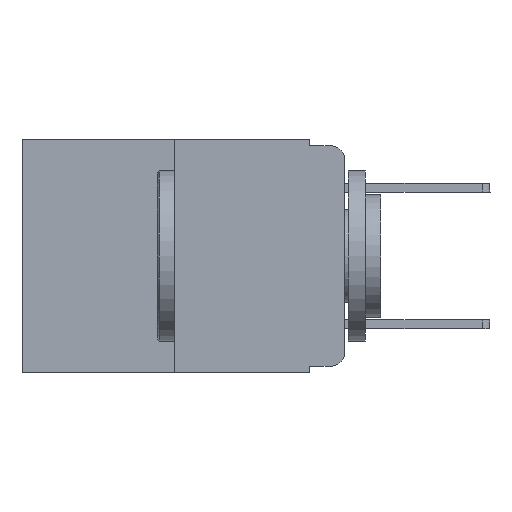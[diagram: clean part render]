
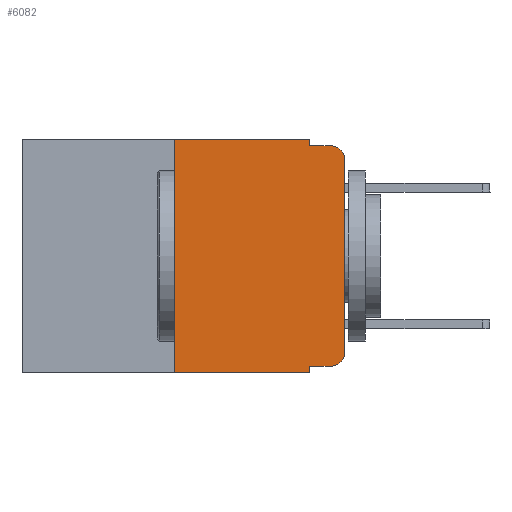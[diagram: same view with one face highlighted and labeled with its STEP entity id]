
A CAD part, left-side view. The second image highlights one B-rep face of the part: STEP entity #6082.
In plain terms, the highlighted planar face has unit normal (-1, 0, 0).
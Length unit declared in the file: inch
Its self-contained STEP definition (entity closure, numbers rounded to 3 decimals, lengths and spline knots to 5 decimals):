
#57 = VECTOR ( 'NONE', #6023, 39.37008 ) ;
#401 = FACE_OUTER_BOUND ( 'NONE', #14951, .T. ) ;
#591 = ORIENTED_EDGE ( 'NONE', *, *, #9521, .F. ) ;
#711 = VECTOR ( 'NONE', #925, 39.37008 ) ;
#925 = DIRECTION ( 'NONE',  ( 0., 0., -1. ) ) ;
#1320 = VECTOR ( 'NONE', #15416, 39.37008 ) ;
#1737 = VECTOR ( 'NONE', #19140, 39.37008 ) ;
#1847 = LINE ( 'NONE', #5920, #57 ) ;
#2162 = DIRECTION ( 'NONE',  ( 0., -1., 0. ) ) ;
#2220 = VERTEX_POINT ( 'NONE', #3513 ) ;
#2320 = LINE ( 'NONE', #8264, #16918 ) ;
#2785 = VERTEX_POINT ( 'NONE', #6773 ) ;
#2988 = CIRCLE ( 'NONE', #18828, 0.02 ) ;
#3513 = CARTESIAN_POINT ( 'NONE',  ( 0., 0.051, 0. ) ) ;
#3861 = CARTESIAN_POINT ( 'NONE',  ( 0., 0.051, 0. ) ) ;
#4097 = ORIENTED_EDGE ( 'NONE', *, *, #16915, .F. ) ;
#4651 = VERTEX_POINT ( 'NONE', #17938 ) ;
#4690 = DIRECTION ( 'NONE',  ( 1., 0., 0. ) ) ;
#4806 = EDGE_CURVE ( 'NONE', #4651, #12402, #2320, .T. ) ;
#4837 = AXIS2_PLACEMENT_3D ( 'NONE', #6353, #4690, #6451 ) ;
#5511 = DIRECTION ( 'NONE',  ( 0., 0., -1. ) ) ;
#5723 = VERTEX_POINT ( 'NONE', #9205 ) ;
#5794 = CARTESIAN_POINT ( 'NONE',  ( 0., 0., 0. ) ) ;
#5920 = CARTESIAN_POINT ( 'NONE',  ( 0., 0.051, 0. ) ) ;
#6023 = DIRECTION ( 'NONE',  ( 0., 0., -1. ) ) ;
#6063 = VECTOR ( 'NONE', #2162, 39.37008 ) ;
#6082 = ADVANCED_FACE ( 'NONE', ( #401 ), #6254, .F. ) ;
#6254 = PLANE ( 'NONE',  #4837 ) ;
#6353 = CARTESIAN_POINT ( 'NONE',  ( 0., 0.473, 0. ) ) ;
#6374 = DIRECTION ( 'NONE',  ( 0., -1., 0. ) ) ;
#6451 = DIRECTION ( 'NONE',  ( 0., 0., -1. ) ) ;
#6548 = ORIENTED_EDGE ( 'NONE', *, *, #11520, .F. ) ;
#6652 = LINE ( 'NONE', #18429, #1320 ) ;
#6667 = DIRECTION ( 'NONE',  ( 0., 0., 1. ) ) ;
#6773 = CARTESIAN_POINT ( 'NONE',  ( 0., 0.25, 0. ) ) ;
#6784 = CARTESIAN_POINT ( 'NONE',  ( 0., 0., -0.03 ) ) ;
#6912 = AXIS2_PLACEMENT_3D ( 'NONE', #16498, #12036, #12140 ) ;
#7040 = ORIENTED_EDGE ( 'NONE', *, *, #15176, .T. ) ;
#7528 = VERTEX_POINT ( 'NONE', #17605 ) ;
#7849 = ORIENTED_EDGE ( 'NONE', *, *, #14947, .F. ) ;
#8008 = VECTOR ( 'NONE', #6667, 39.37008 ) ;
#8264 = CARTESIAN_POINT ( 'NONE',  ( 0., 0.051, -0.01 ) ) ;
#8389 = CARTESIAN_POINT ( 'NONE',  ( 0., 0.02, -0.333 ) ) ;
#9041 = VERTEX_POINT ( 'NONE', #6784 ) ;
#9205 = CARTESIAN_POINT ( 'NONE',  ( 0., 0.051, -0.343 ) ) ;
#9217 = EDGE_CURVE ( 'NONE', #9041, #12402, #2988, .T. ) ;
#9238 = EDGE_CURVE ( 'NONE', #7528, #9041, #14370, .T. ) ;
#9391 = CARTESIAN_POINT ( 'NONE',  ( 0., 0.473, -0.343 ) ) ;
#9521 = EDGE_CURVE ( 'NONE', #10757, #2785, #13977, .T. ) ;
#9576 = ORIENTED_EDGE ( 'NONE', *, *, #15290, .T. ) ;
#9914 = ORIENTED_EDGE ( 'NONE', *, *, #9217, .T. ) ;
#10207 = CARTESIAN_POINT ( 'NONE',  ( 0., 0.051, -0.333 ) ) ;
#10757 = VERTEX_POINT ( 'NONE', #15527 ) ;
#11257 = LINE ( 'NONE', #3861, #711 ) ;
#11443 = CARTESIAN_POINT ( 'NONE',  ( 0., 0.02, -0.01 ) ) ;
#11520 = EDGE_CURVE ( 'NONE', #2220, #4651, #1847, .T. ) ;
#12036 = DIRECTION ( 'NONE',  ( -1., 0., 0. ) ) ;
#12140 = DIRECTION ( 'NONE',  ( 0., 0., -1. ) ) ;
#12395 = LINE ( 'NONE', #16671, #6063 ) ;
#12402 = VERTEX_POINT ( 'NONE', #11443 ) ;
#13196 = VERTEX_POINT ( 'NONE', #10207 ) ;
#13207 = CARTESIAN_POINT ( 'NONE',  ( 0., 0.02, -0.03 ) ) ;
#13977 = LINE ( 'NONE', #15613, #8008 ) ;
#14195 = DIRECTION ( 'NONE',  ( 0., -1., 0. ) ) ;
#14370 = LINE ( 'NONE', #5794, #1737 ) ;
#14561 = VERTEX_POINT ( 'NONE', #8389 ) ;
#14947 = EDGE_CURVE ( 'NONE', #13196, #5723, #11257, .T. ) ;
#14951 = EDGE_LOOP ( 'NONE', ( #17438, #9914, #16512, #6548, #4097, #591, #18533, #7849, #9576, #7040 ) ) ;
#15176 = EDGE_CURVE ( 'NONE', #14561, #7528, #19052, .T. ) ;
#15290 = EDGE_CURVE ( 'NONE', #13196, #14561, #6652, .T. ) ;
#15326 = LINE ( 'NONE', #9391, #15420 ) ;
#15416 = DIRECTION ( 'NONE',  ( 0., -1., 0. ) ) ;
#15420 = VECTOR ( 'NONE', #6374, 39.37008 ) ;
#15527 = CARTESIAN_POINT ( 'NONE',  ( 0., 0.25, -0.343 ) ) ;
#15613 = CARTESIAN_POINT ( 'NONE',  ( 0., 0.25, 0. ) ) ;
#16498 = CARTESIAN_POINT ( 'NONE',  ( 0., 0.02, -0.313 ) ) ;
#16512 = ORIENTED_EDGE ( 'NONE', *, *, #4806, .F. ) ;
#16671 = CARTESIAN_POINT ( 'NONE',  ( 0., 0.473, 0. ) ) ;
#16915 = EDGE_CURVE ( 'NONE', #2785, #2220, #12395, .T. ) ;
#16918 = VECTOR ( 'NONE', #14195, 39.37008 ) ;
#17438 = ORIENTED_EDGE ( 'NONE', *, *, #9238, .T. ) ;
#17585 = DIRECTION ( 'NONE',  ( -1., 0., 0. ) ) ;
#17605 = CARTESIAN_POINT ( 'NONE',  ( 0., 0., -0.313 ) ) ;
#17938 = CARTESIAN_POINT ( 'NONE',  ( 0., 0.051, -0.01 ) ) ;
#18155 = EDGE_CURVE ( 'NONE', #10757, #5723, #15326, .T. ) ;
#18429 = CARTESIAN_POINT ( 'NONE',  ( 0., 0.051, -0.333 ) ) ;
#18533 = ORIENTED_EDGE ( 'NONE', *, *, #18155, .T. ) ;
#18828 = AXIS2_PLACEMENT_3D ( 'NONE', #13207, #17585, #5511 ) ;
#19052 = CIRCLE ( 'NONE', #6912, 0.02 ) ;
#19140 = DIRECTION ( 'NONE',  ( 0., 0., 1. ) ) ;
